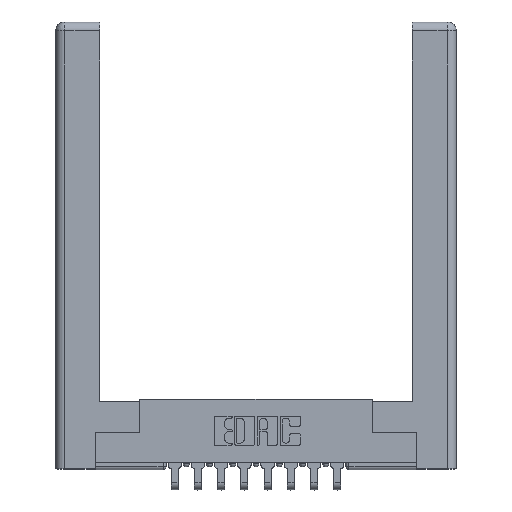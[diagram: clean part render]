
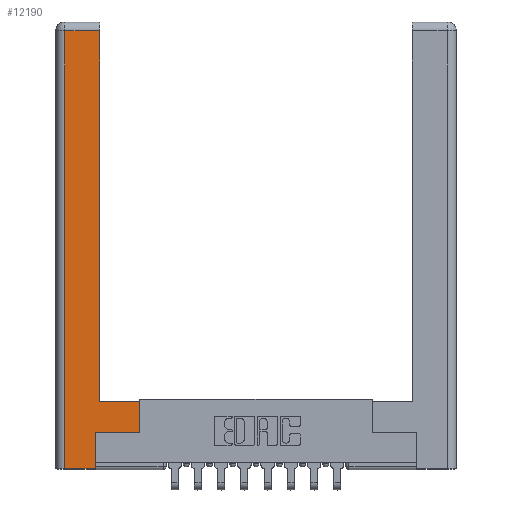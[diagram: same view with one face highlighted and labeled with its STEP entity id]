
A CAD part, top view. The second image highlights one B-rep face of the part: STEP entity #12190.
In plain terms, the highlighted planar face has unit normal (0, 0, 1).
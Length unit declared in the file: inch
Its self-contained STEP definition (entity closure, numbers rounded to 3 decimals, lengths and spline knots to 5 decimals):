
#873 = VECTOR ( 'NONE', #10962, 39.37008 ) ;
#1045 = CARTESIAN_POINT ( 'NONE',  ( 0.0615, 2.94, 0. ) ) ;
#1123 = VECTOR ( 'NONE', #5994, 39.37008 ) ;
#1244 = EDGE_CURVE ( 'NONE', #8714, #10004, #3670, .T. ) ;
#1346 = ORIENTED_EDGE ( 'NONE', *, *, #5960, .T. ) ;
#1788 = ORIENTED_EDGE ( 'NONE', *, *, #10354, .T. ) ;
#1818 = FACE_OUTER_BOUND ( 'NONE', #8579, .T. ) ;
#1831 = VERTEX_POINT ( 'NONE', #5109 ) ;
#2102 = AXIS2_PLACEMENT_3D ( 'NONE', #5370, #4341, #11979 ) ;
#2243 = CARTESIAN_POINT ( 'NONE',  ( 0.565, 0.45, 0. ) ) ;
#2351 = VERTEX_POINT ( 'NONE', #9167 ) ;
#2612 = VECTOR ( 'NONE', #8570, 39.37008 ) ;
#2931 = CARTESIAN_POINT ( 'NONE',  ( 0.565, 0.245, 0. ) ) ;
#3388 = CARTESIAN_POINT ( 'NONE',  ( 0.295, 0.45, 0. ) ) ;
#3472 = EDGE_CURVE ( 'NONE', #11613, #1831, #13273, .T. ) ;
#3670 = LINE ( 'NONE', #2243, #10835 ) ;
#3792 = CARTESIAN_POINT ( 'NONE',  ( 0.295, 3., 0. ) ) ;
#3908 = CARTESIAN_POINT ( 'NONE',  ( 0.265, 0.245, 0. ) ) ;
#4341 = DIRECTION ( 'NONE',  ( 0., 0., -1. ) ) ;
#4470 = LINE ( 'NONE', #3388, #2612 ) ;
#4655 = ORIENTED_EDGE ( 'NONE', *, *, #13074, .T. ) ;
#4736 = LINE ( 'NONE', #3908, #5225 ) ;
#4783 = ORIENTED_EDGE ( 'NONE', *, *, #10351, .T. ) ;
#5109 = CARTESIAN_POINT ( 'NONE',  ( 0.295, 2.94, 0. ) ) ;
#5225 = VECTOR ( 'NONE', #13622, 39.37008 ) ;
#5370 = CARTESIAN_POINT ( 'NONE',  ( 0., 0., 0. ) ) ;
#5845 = CARTESIAN_POINT ( 'NONE',  ( 0.265, 0.245, 0. ) ) ;
#5960 = EDGE_CURVE ( 'NONE', #13316, #7011, #10067, .T. ) ;
#5994 = DIRECTION ( 'NONE',  ( -1., 0., 0. ) ) ;
#6574 = DIRECTION ( 'NONE',  ( 0., 1., 0. ) ) ;
#6802 = ORIENTED_EDGE ( 'NONE', *, *, #13368, .T. ) ;
#7011 = VERTEX_POINT ( 'NONE', #10432 ) ;
#7409 = VECTOR ( 'NONE', #11280, 39.37008 ) ;
#8197 = CARTESIAN_POINT ( 'NONE',  ( 0.0615, 2.94, 0. ) ) ;
#8473 = CARTESIAN_POINT ( 'NONE',  ( 0.565, 0.245, 0. ) ) ;
#8570 = DIRECTION ( 'NONE',  ( -1., 0., 0. ) ) ;
#8579 = EDGE_LOOP ( 'NONE', ( #11515, #4655, #1346, #4783, #1788, #10173, #12381, #6802 ) ) ;
#8714 = VERTEX_POINT ( 'NONE', #2931 ) ;
#8736 = CARTESIAN_POINT ( 'NONE',  ( 0.565, 0.45, 0. ) ) ;
#9167 = CARTESIAN_POINT ( 'NONE',  ( 0.265, 0., 0. ) ) ;
#9190 = CARTESIAN_POINT ( 'NONE',  ( 0.295, 0.45, 0. ) ) ;
#9551 = VERTEX_POINT ( 'NONE', #5845 ) ;
#10004 = VERTEX_POINT ( 'NONE', #8736 ) ;
#10067 = LINE ( 'NONE', #12068, #873 ) ;
#10112 = VECTOR ( 'NONE', #13471, 39.37008 ) ;
#10173 = ORIENTED_EDGE ( 'NONE', *, *, #10548, .T. ) ;
#10218 = VECTOR ( 'NONE', #10568, 39.37008 ) ;
#10351 = EDGE_CURVE ( 'NONE', #7011, #2351, #13222, .T. ) ;
#10354 = EDGE_CURVE ( 'NONE', #2351, #9551, #4736, .T. ) ;
#10432 = CARTESIAN_POINT ( 'NONE',  ( 0.0615, 0., 0. ) ) ;
#10548 = EDGE_CURVE ( 'NONE', #9551, #8714, #11545, .T. ) ;
#10568 = DIRECTION ( 'NONE',  ( 1., 0., 0. ) ) ;
#10835 = VECTOR ( 'NONE', #6574, 39.37008 ) ;
#10962 = DIRECTION ( 'NONE',  ( 0., -1., 0. ) ) ;
#11280 = DIRECTION ( 'NONE',  ( 1., 0., 0. ) ) ;
#11515 = ORIENTED_EDGE ( 'NONE', *, *, #3472, .T. ) ;
#11545 = LINE ( 'NONE', #8473, #10218 ) ;
#11613 = VERTEX_POINT ( 'NONE', #9190 ) ;
#11746 = PLANE ( 'NONE',  #2102 ) ;
#11979 = DIRECTION ( 'NONE',  ( -1., 0., 0. ) ) ;
#12068 = CARTESIAN_POINT ( 'NONE',  ( 0.0615, 0., 0. ) ) ;
#12190 = ADVANCED_FACE ( 'NONE', ( #1818 ), #11746, .F. ) ;
#12381 = ORIENTED_EDGE ( 'NONE', *, *, #1244, .T. ) ;
#13074 = EDGE_CURVE ( 'NONE', #1831, #13316, #13782, .T. ) ;
#13222 = LINE ( 'NONE', #13402, #7409 ) ;
#13273 = LINE ( 'NONE', #3792, #10112 ) ;
#13316 = VERTEX_POINT ( 'NONE', #1045 ) ;
#13368 = EDGE_CURVE ( 'NONE', #10004, #11613, #4470, .T. ) ;
#13402 = CARTESIAN_POINT ( 'NONE',  ( 0.265, 0., 0. ) ) ;
#13471 = DIRECTION ( 'NONE',  ( 0., 1., 0. ) ) ;
#13622 = DIRECTION ( 'NONE',  ( 0., 1., 0. ) ) ;
#13782 = LINE ( 'NONE', #8197, #1123 ) ;
